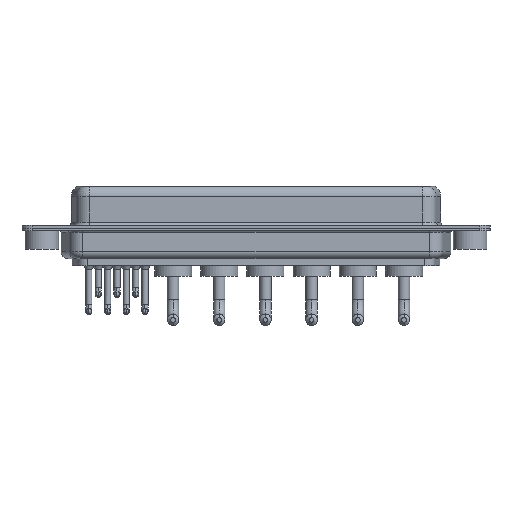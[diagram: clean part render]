
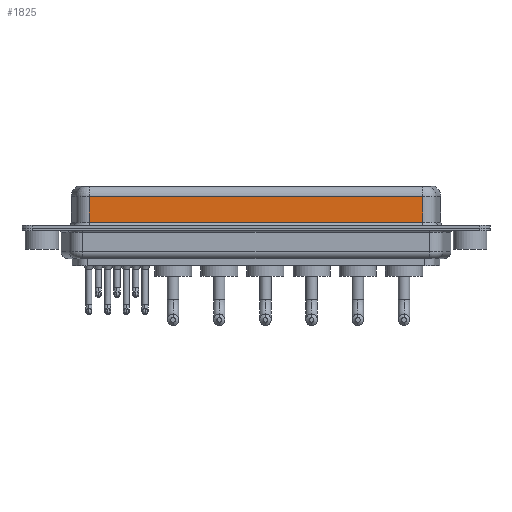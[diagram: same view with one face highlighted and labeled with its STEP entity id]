
A CAD part, front view. The second image highlights one B-rep face of the part: STEP entity #1825.
In plain terms, the highlighted planar face has unit normal (0, -1, 0).
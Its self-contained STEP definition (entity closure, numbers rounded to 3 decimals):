
#1059 = EDGE_LOOP ( 'NONE', ( #5999, #3655, #7764, #14493 ) ) ;
#1232 = VECTOR ( 'NONE', #15807, 1000. ) ;
#1647 = CARTESIAN_POINT ( 'NONE',  ( 56.462, -3.95, 4.65 ) ) ;
#1825 = ADVANCED_FACE ( 'NONE', ( #7553 ), #6420, .F. ) ;
#1951 = VERTEX_POINT ( 'NONE', #17076 ) ;
#2023 = DIRECTION ( 'NONE',  ( 0., 0., 1. ) ) ;
#3130 = DIRECTION ( 'NONE',  ( 0., 0., -1. ) ) ;
#3655 = ORIENTED_EDGE ( 'NONE', *, *, #7856, .T. ) ;
#4835 = CARTESIAN_POINT ( 'NONE',  ( 56.462, -3.95, 6.4 ) ) ;
#5811 = LINE ( 'NONE', #9856, #1232 ) ;
#5968 = VERTEX_POINT ( 'NONE', #8979 ) ;
#5999 = ORIENTED_EDGE ( 'NONE', *, *, #6361, .F. ) ;
#6361 = EDGE_CURVE ( 'NONE', #7788, #18119, #13367, .T. ) ;
#6420 = PLANE ( 'NONE',  #8904 ) ;
#6468 = EDGE_CURVE ( 'NONE', #1951, #18119, #5811, .T. ) ;
#7344 = DIRECTION ( 'NONE',  ( -1., 0., 0. ) ) ;
#7553 = FACE_OUTER_BOUND ( 'NONE', #1059, .T. ) ;
#7764 = ORIENTED_EDGE ( 'NONE', *, *, #18325, .T. ) ;
#7788 = VERTEX_POINT ( 'NONE', #8466 ) ;
#7856 = EDGE_CURVE ( 'NONE', #7788, #5968, #14427, .T. ) ;
#8466 = CARTESIAN_POINT ( 'NONE',  ( 56.462, -3.95, 4.65 ) ) ;
#8904 = AXIS2_PLACEMENT_3D ( 'NONE', #4835, #14809, #2023 ) ;
#8979 = CARTESIAN_POINT ( 'NONE',  ( 7.038, -3.95, 4.65 ) ) ;
#9856 = CARTESIAN_POINT ( 'NONE',  ( 56.462, -3.95, 0.9 ) ) ;
#12694 = VECTOR ( 'NONE', #3130, 1000. ) ;
#13367 = LINE ( 'NONE', #14686, #12694 ) ;
#13514 = LINE ( 'NONE', #13787, #16342 ) ;
#13787 = CARTESIAN_POINT ( 'NONE',  ( 7.038, -3.95, 6.4 ) ) ;
#14241 = CARTESIAN_POINT ( 'NONE',  ( 56.462, -3.95, 0.9 ) ) ;
#14427 = LINE ( 'NONE', #1647, #15114 ) ;
#14493 = ORIENTED_EDGE ( 'NONE', *, *, #6468, .T. ) ;
#14686 = CARTESIAN_POINT ( 'NONE',  ( 56.462, -3.95, 6.4 ) ) ;
#14809 = DIRECTION ( 'NONE',  ( 0., 1., 0. ) ) ;
#15114 = VECTOR ( 'NONE', #7344, 1000. ) ;
#15807 = DIRECTION ( 'NONE',  ( 1., 0., 0. ) ) ;
#16342 = VECTOR ( 'NONE', #16514, 1000. ) ;
#16514 = DIRECTION ( 'NONE',  ( 0., 0., -1. ) ) ;
#17076 = CARTESIAN_POINT ( 'NONE',  ( 7.038, -3.95, 0.9 ) ) ;
#18119 = VERTEX_POINT ( 'NONE', #14241 ) ;
#18325 = EDGE_CURVE ( 'NONE', #5968, #1951, #13514, .T. ) ;
